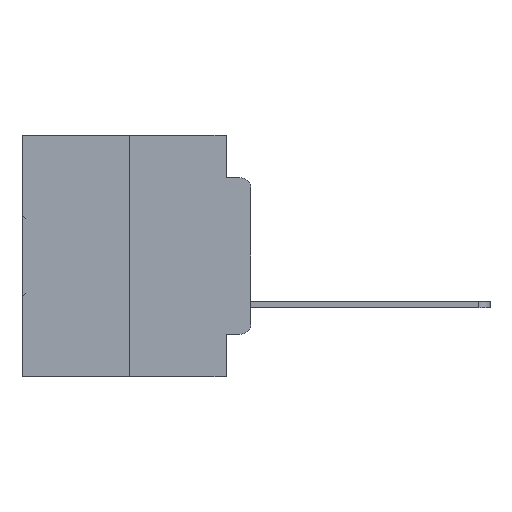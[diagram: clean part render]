
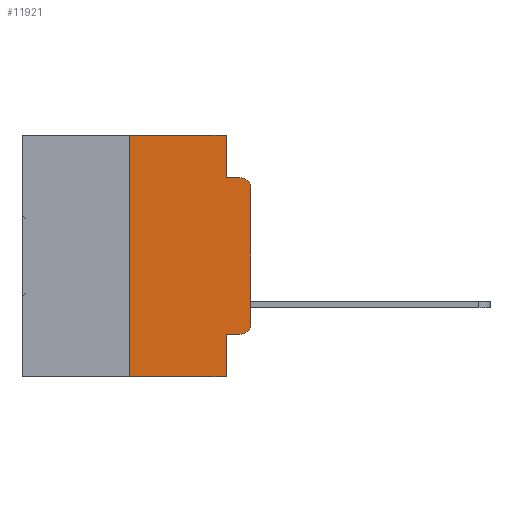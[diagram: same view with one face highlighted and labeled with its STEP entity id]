
A CAD part, left-side view. The second image highlights one B-rep face of the part: STEP entity #11921.
In plain terms, the highlighted planar face has unit normal (-1, 0, 0).
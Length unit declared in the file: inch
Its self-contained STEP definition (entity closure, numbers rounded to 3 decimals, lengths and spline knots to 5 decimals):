
#135 = DIRECTION ( 'NONE',  ( 0., -1., 0. ) ) ;
#349 = VERTEX_POINT ( 'NONE', #9026 ) ;
#466 = LINE ( 'NONE', #27014, #10218 ) ;
#652 = DIRECTION ( 'NONE',  ( 0., 0., -1. ) ) ;
#1012 = CARTESIAN_POINT ( 'NONE',  ( 0., 0.473, 0. ) ) ;
#1449 = VECTOR ( 'NONE', #12522, 39.37008 ) ;
#2265 = AXIS2_PLACEMENT_3D ( 'NONE', #34103, #26134, #32496 ) ;
#2270 = DIRECTION ( 'NONE',  ( 0., 0., -1. ) ) ;
#2627 = LINE ( 'NONE', #30055, #18072 ) ;
#3324 = CARTESIAN_POINT ( 'NONE',  ( 0., 0.051, -0.0885 ) ) ;
#4394 = LINE ( 'NONE', #17469, #5216 ) ;
#4740 = CARTESIAN_POINT ( 'NONE',  ( 0., 0.25, 0. ) ) ;
#5216 = VECTOR ( 'NONE', #28102, 39.37008 ) ;
#5376 = VERTEX_POINT ( 'NONE', #16301 ) ;
#6897 = EDGE_CURVE ( 'NONE', #11380, #21733, #32773, .T. ) ;
#7692 = VERTEX_POINT ( 'NONE', #15714 ) ;
#8988 = PLANE ( 'NONE',  #29938 ) ;
#9026 = CARTESIAN_POINT ( 'NONE',  ( 0., 0., -0.3915 ) ) ;
#9241 = VECTOR ( 'NONE', #2270, 39.37008 ) ;
#9815 = CARTESIAN_POINT ( 'NONE',  ( 0., 0.051, 0. ) ) ;
#10001 = VECTOR ( 'NONE', #20213, 39.37008 ) ;
#10218 = VECTOR ( 'NONE', #30045, 39.37008 ) ;
#11217 = CARTESIAN_POINT ( 'NONE',  ( 0., 0.25, 0. ) ) ;
#11380 = VERTEX_POINT ( 'NONE', #21570 ) ;
#11758 = EDGE_CURVE ( 'NONE', #29690, #19326, #466, .T. ) ;
#11847 = VERTEX_POINT ( 'NONE', #30754 ) ;
#11921 = ADVANCED_FACE ( 'NONE', ( #25407 ), #8988, .F. ) ;
#12522 = DIRECTION ( 'NONE',  ( 0., 0., 1. ) ) ;
#12905 = EDGE_CURVE ( 'NONE', #16539, #29690, #2627, .T. ) ;
#13772 = LINE ( 'NONE', #24554, #22871 ) ;
#13971 = ORIENTED_EDGE ( 'NONE', *, *, #17186, .F. ) ;
#14741 = VERTEX_POINT ( 'NONE', #27853 ) ;
#14981 = EDGE_CURVE ( 'NONE', #349, #11380, #31732, .T. ) ;
#15157 = CIRCLE ( 'NONE', #34933, 0.02 ) ;
#15714 = CARTESIAN_POINT ( 'NONE',  ( 0., 0.051, -0.4115 ) ) ;
#15815 = CARTESIAN_POINT ( 'NONE',  ( 0., 0.02, -0.3915 ) ) ;
#15884 = CARTESIAN_POINT ( 'NONE',  ( 0., 0.02, -0.0885 ) ) ;
#16301 = CARTESIAN_POINT ( 'NONE',  ( 0., 0.051, -0.5 ) ) ;
#16436 = ORIENTED_EDGE ( 'NONE', *, *, #31830, .T. ) ;
#16539 = VERTEX_POINT ( 'NONE', #11217 ) ;
#17186 = EDGE_CURVE ( 'NONE', #7692, #5376, #21344, .T. ) ;
#17469 = CARTESIAN_POINT ( 'NONE',  ( 0., 0.051, -0.4115 ) ) ;
#17809 = LINE ( 'NONE', #4740, #1449 ) ;
#18072 = VECTOR ( 'NONE', #135, 39.37008 ) ;
#18383 = DIRECTION ( 'NONE',  ( 0., -1., 0. ) ) ;
#19006 = DIRECTION ( 'NONE',  ( -1., 0., 0. ) ) ;
#19326 = VERTEX_POINT ( 'NONE', #3324 ) ;
#20213 = DIRECTION ( 'NONE',  ( 0., -1., 0. ) ) ;
#20455 = EDGE_CURVE ( 'NONE', #11847, #5376, #13772, .T. ) ;
#20772 = EDGE_CURVE ( 'NONE', #11847, #16539, #17809, .T. ) ;
#21344 = LINE ( 'NONE', #32163, #9241 ) ;
#21570 = CARTESIAN_POINT ( 'NONE',  ( 0., 0., -0.1085 ) ) ;
#21733 = VERTEX_POINT ( 'NONE', #15884 ) ;
#21901 = ORIENTED_EDGE ( 'NONE', *, *, #6897, .T. ) ;
#22871 = VECTOR ( 'NONE', #18383, 39.37008 ) ;
#24125 = ORIENTED_EDGE ( 'NONE', *, *, #20772, .F. ) ;
#24554 = CARTESIAN_POINT ( 'NONE',  ( 0., 0.473, -0.5 ) ) ;
#24727 = EDGE_CURVE ( 'NONE', #19326, #21733, #25886, .T. ) ;
#24889 = DIRECTION ( 'NONE',  ( 1., 0., 0. ) ) ;
#25014 = ORIENTED_EDGE ( 'NONE', *, *, #20455, .T. ) ;
#25407 = FACE_OUTER_BOUND ( 'NONE', #28323, .T. ) ;
#25527 = CARTESIAN_POINT ( 'NONE',  ( 0., 0., 0. ) ) ;
#25886 = LINE ( 'NONE', #26059, #10001 ) ;
#26059 = CARTESIAN_POINT ( 'NONE',  ( 0., 0.051, -0.0885 ) ) ;
#26091 = ORIENTED_EDGE ( 'NONE', *, *, #28170, .T. ) ;
#26134 = DIRECTION ( 'NONE',  ( -1., 0., 0. ) ) ;
#26230 = DIRECTION ( 'NONE',  ( 0., 0., 1. ) ) ;
#27014 = CARTESIAN_POINT ( 'NONE',  ( 0., 0.051, 0. ) ) ;
#27818 = ORIENTED_EDGE ( 'NONE', *, *, #12905, .F. ) ;
#27853 = CARTESIAN_POINT ( 'NONE',  ( 0., 0.02, -0.4115 ) ) ;
#28102 = DIRECTION ( 'NONE',  ( 0., -1., 0. ) ) ;
#28170 = EDGE_CURVE ( 'NONE', #14741, #349, #15157, .T. ) ;
#28323 = EDGE_LOOP ( 'NONE', ( #32348, #21901, #28479, #30771, #27818, #24125, #25014, #13971, #16436, #26091 ) ) ;
#28479 = ORIENTED_EDGE ( 'NONE', *, *, #24727, .F. ) ;
#29690 = VERTEX_POINT ( 'NONE', #9815 ) ;
#29938 = AXIS2_PLACEMENT_3D ( 'NONE', #1012, #24889, #652 ) ;
#30045 = DIRECTION ( 'NONE',  ( 0., 0., -1. ) ) ;
#30055 = CARTESIAN_POINT ( 'NONE',  ( 0., 0.473, 0. ) ) ;
#30754 = CARTESIAN_POINT ( 'NONE',  ( 0., 0.25, -0.5 ) ) ;
#30771 = ORIENTED_EDGE ( 'NONE', *, *, #11758, .F. ) ;
#31732 = LINE ( 'NONE', #25527, #34533 ) ;
#31830 = EDGE_CURVE ( 'NONE', #7692, #14741, #4394, .T. ) ;
#32163 = CARTESIAN_POINT ( 'NONE',  ( 0., 0.051, 0. ) ) ;
#32348 = ORIENTED_EDGE ( 'NONE', *, *, #14981, .T. ) ;
#32496 = DIRECTION ( 'NONE',  ( 0., 0., -1. ) ) ;
#32647 = DIRECTION ( 'NONE',  ( 0., 0., -1. ) ) ;
#32773 = CIRCLE ( 'NONE', #2265, 0.02 ) ;
#34103 = CARTESIAN_POINT ( 'NONE',  ( 0., 0.02, -0.1085 ) ) ;
#34533 = VECTOR ( 'NONE', #26230, 39.37008 ) ;
#34933 = AXIS2_PLACEMENT_3D ( 'NONE', #15815, #19006, #32647 ) ;
